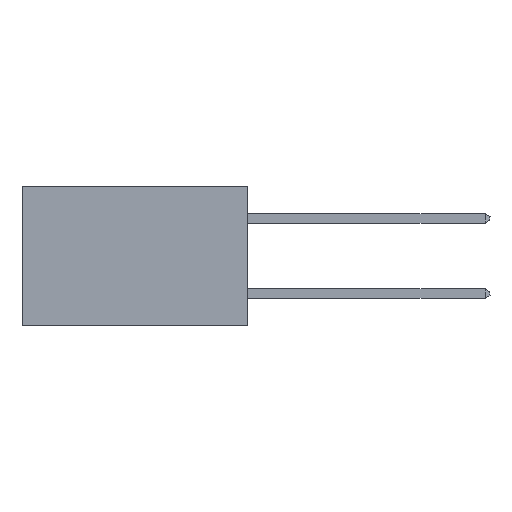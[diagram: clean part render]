
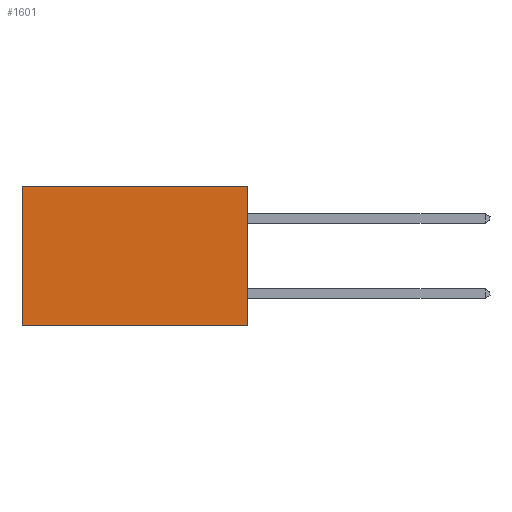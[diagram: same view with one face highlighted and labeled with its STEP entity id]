
A CAD part, left-side view. The second image highlights one B-rep face of the part: STEP entity #1601.
In plain terms, the highlighted planar face has unit normal (-1, 0, 0).
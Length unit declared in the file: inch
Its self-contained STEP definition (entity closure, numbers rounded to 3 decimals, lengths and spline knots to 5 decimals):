
#123 = EDGE_LOOP ( 'NONE', ( #8062, #8715, #8185, #3786 ) ) ;
#217 = CARTESIAN_POINT ( 'NONE',  ( 0.298, 0., 0. ) ) ;
#577 = DIRECTION ( 'NONE',  ( 0., 1., 0. ) ) ;
#924 = LINE ( 'NONE', #217, #4210 ) ;
#1104 = DIRECTION ( 'NONE',  ( 0., 0., -1. ) ) ;
#1296 = CARTESIAN_POINT ( 'NONE',  ( 0.298, 0., 0. ) ) ;
#1601 = ADVANCED_FACE ( 'NONE', ( #3516 ), #2828, .F. ) ;
#1659 = DIRECTION ( 'NONE',  ( 0., 0., -1. ) ) ;
#2828 = PLANE ( 'NONE',  #6002 ) ;
#3070 = CARTESIAN_POINT ( 'NONE',  ( 0.298, 0.6, -0.37 ) ) ;
#3347 = CARTESIAN_POINT ( 'NONE',  ( 0.298, 0., -0.37 ) ) ;
#3448 = EDGE_CURVE ( 'NONE', #6258, #7543, #7355, .T. ) ;
#3516 = FACE_OUTER_BOUND ( 'NONE', #123, .T. ) ;
#3673 = VECTOR ( 'NONE', #577, 39.37008 ) ;
#3769 = DIRECTION ( 'NONE',  ( 0., 1., 0. ) ) ;
#3786 = ORIENTED_EDGE ( 'NONE', *, *, #5986, .T. ) ;
#4051 = VECTOR ( 'NONE', #3769, 39.37008 ) ;
#4169 = CARTESIAN_POINT ( 'NONE',  ( 0.298, 0., 0. ) ) ;
#4210 = VECTOR ( 'NONE', #1659, 39.37008 ) ;
#4968 = CARTESIAN_POINT ( 'NONE',  ( 0.298, 0.6, 0. ) ) ;
#5259 = EDGE_CURVE ( 'NONE', #5511, #6258, #924, .T. ) ;
#5511 = VERTEX_POINT ( 'NONE', #1296 ) ;
#5615 = DIRECTION ( 'NONE',  ( 1., 0., 0. ) ) ;
#5986 = EDGE_CURVE ( 'NONE', #5511, #8950, #8504, .T. ) ;
#6002 = AXIS2_PLACEMENT_3D ( 'NONE', #4169, #5615, #6235 ) ;
#6088 = VECTOR ( 'NONE', #1104, 39.37008 ) ;
#6235 = DIRECTION ( 'NONE',  ( 0., 0., -1. ) ) ;
#6258 = VERTEX_POINT ( 'NONE', #3347 ) ;
#6617 = CARTESIAN_POINT ( 'NONE',  ( 0.298, 0.6, 0. ) ) ;
#6642 = EDGE_CURVE ( 'NONE', #8950, #7543, #8279, .T. ) ;
#6935 = CARTESIAN_POINT ( 'NONE',  ( 0.298, 0., -0.37 ) ) ;
#7355 = LINE ( 'NONE', #6935, #3673 ) ;
#7543 = VERTEX_POINT ( 'NONE', #3070 ) ;
#7936 = CARTESIAN_POINT ( 'NONE',  ( 0.298, 0., 0. ) ) ;
#8062 = ORIENTED_EDGE ( 'NONE', *, *, #6642, .T. ) ;
#8185 = ORIENTED_EDGE ( 'NONE', *, *, #5259, .F. ) ;
#8279 = LINE ( 'NONE', #6617, #6088 ) ;
#8504 = LINE ( 'NONE', #7936, #4051 ) ;
#8715 = ORIENTED_EDGE ( 'NONE', *, *, #3448, .F. ) ;
#8950 = VERTEX_POINT ( 'NONE', #4968 ) ;
